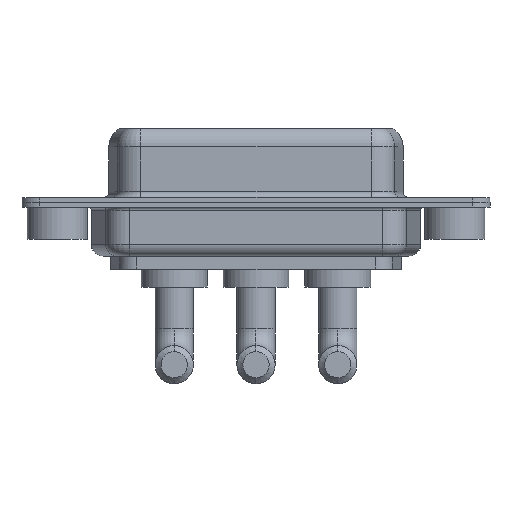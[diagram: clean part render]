
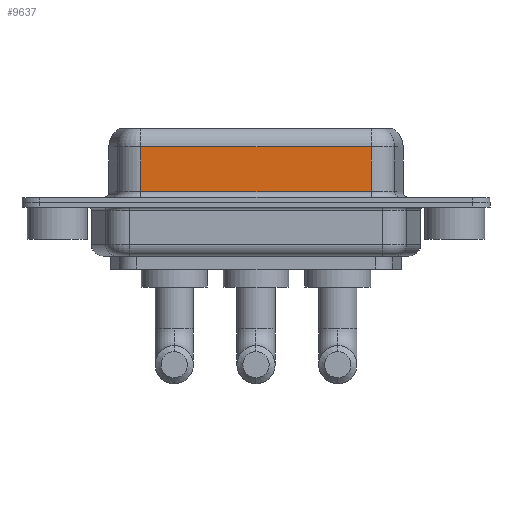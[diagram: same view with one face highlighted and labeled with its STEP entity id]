
A CAD part, front view. The second image highlights one B-rep face of the part: STEP entity #9637.
In plain terms, the highlighted planar face has unit normal (0, -1, 0).
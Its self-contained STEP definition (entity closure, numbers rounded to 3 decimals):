
#90 = DIRECTION ( 'NONE',  ( 0., 1., 0. ) ) ;
#2384 = ORIENTED_EDGE ( 'NONE', *, *, #4933, .T. ) ;
#2948 = VECTOR ( 'NONE', #4770, 1000. ) ;
#3131 = CARTESIAN_POINT ( 'NONE',  ( 26.287, -3.95, 4.65 ) ) ;
#3496 = LINE ( 'NONE', #7305, #5090 ) ;
#3506 = FACE_OUTER_BOUND ( 'NONE', #3731, .T. ) ;
#3731 = EDGE_LOOP ( 'NONE', ( #4486, #4473, #7725, #2384 ) ) ;
#4473 = ORIENTED_EDGE ( 'NONE', *, *, #5178, .T. ) ;
#4486 = ORIENTED_EDGE ( 'NONE', *, *, #9139, .F. ) ;
#4770 = DIRECTION ( 'NONE',  ( 1., 0., 0. ) ) ;
#4933 = EDGE_CURVE ( 'NONE', #6356, #11279, #9389, .T. ) ;
#5090 = VECTOR ( 'NONE', #10182, 1000. ) ;
#5178 = EDGE_CURVE ( 'NONE', #5566, #8225, #7947, .T. ) ;
#5566 = VERTEX_POINT ( 'NONE', #9554 ) ;
#5593 = CARTESIAN_POINT ( 'NONE',  ( 26.287, -3.95, 6.4 ) ) ;
#6356 = VERTEX_POINT ( 'NONE', #9092 ) ;
#6518 = LINE ( 'NONE', #5593, #10804 ) ;
#7305 = CARTESIAN_POINT ( 'NONE',  ( 7.013, -3.95, 6.4 ) ) ;
#7494 = CARTESIAN_POINT ( 'NONE',  ( 7.013, -3.95, 4.65 ) ) ;
#7725 = ORIENTED_EDGE ( 'NONE', *, *, #11441, .T. ) ;
#7947 = LINE ( 'NONE', #3131, #12353 ) ;
#8225 = VERTEX_POINT ( 'NONE', #7494 ) ;
#8556 = DIRECTION ( 'NONE',  ( 0., 0., 1. ) ) ;
#9052 = CARTESIAN_POINT ( 'NONE',  ( 26.287, -3.95, 0.9 ) ) ;
#9092 = CARTESIAN_POINT ( 'NONE',  ( 7.013, -3.95, 0.9 ) ) ;
#9139 = EDGE_CURVE ( 'NONE', #5566, #11279, #6518, .T. ) ;
#9389 = LINE ( 'NONE', #10574, #2948 ) ;
#9395 = DIRECTION ( 'NONE',  ( 0., 0., -1. ) ) ;
#9554 = CARTESIAN_POINT ( 'NONE',  ( 26.287, -3.95, 4.65 ) ) ;
#9628 = DIRECTION ( 'NONE',  ( -1., 0., 0. ) ) ;
#9637 = ADVANCED_FACE ( 'NONE', ( #3506 ), #11136, .F. ) ;
#10182 = DIRECTION ( 'NONE',  ( 0., 0., -1. ) ) ;
#10574 = CARTESIAN_POINT ( 'NONE',  ( 26.287, -3.95, 0.9 ) ) ;
#10804 = VECTOR ( 'NONE', #9395, 1000. ) ;
#11136 = PLANE ( 'NONE',  #12204 ) ;
#11279 = VERTEX_POINT ( 'NONE', #9052 ) ;
#11441 = EDGE_CURVE ( 'NONE', #8225, #6356, #3496, .T. ) ;
#12018 = CARTESIAN_POINT ( 'NONE',  ( 26.287, -3.95, 6.4 ) ) ;
#12204 = AXIS2_PLACEMENT_3D ( 'NONE', #12018, #90, #8556 ) ;
#12353 = VECTOR ( 'NONE', #9628, 1000. ) ;
